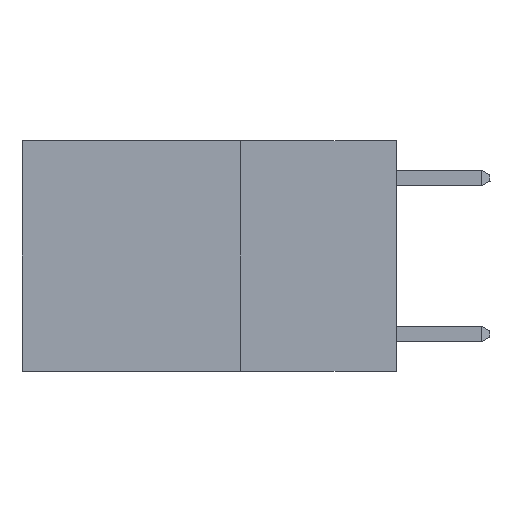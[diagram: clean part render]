
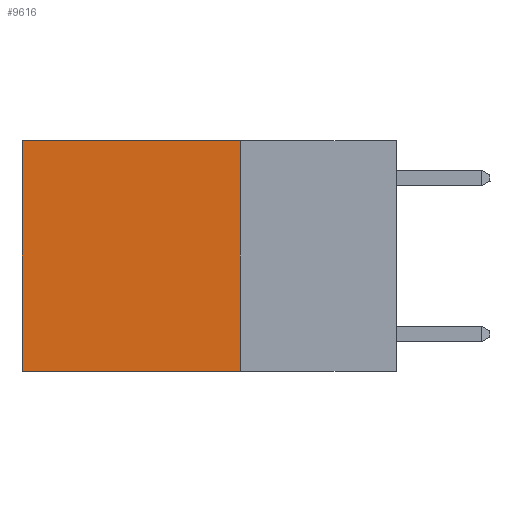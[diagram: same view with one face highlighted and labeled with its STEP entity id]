
A CAD part, left-side view. The second image highlights one B-rep face of the part: STEP entity #9616.
In plain terms, the highlighted planar face has unit normal (-1, 0, 0).
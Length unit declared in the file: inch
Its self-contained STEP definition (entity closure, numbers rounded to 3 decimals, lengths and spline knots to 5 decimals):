
#2076 = VERTEX_POINT ( 'NONE', #5100 ) ;
#2404 = VECTOR ( 'NONE', #7611, 39.37008 ) ;
#2721 = CARTESIAN_POINT ( 'NONE',  ( 0.2625, 0.25, 0. ) ) ;
#4051 = EDGE_CURVE ( 'NONE', #2076, #20402, #18333, .T. ) ;
#4204 = VECTOR ( 'NONE', #20596, 39.37008 ) ;
#4466 = CARTESIAN_POINT ( 'NONE',  ( 0.2625, 0.25, -0.37 ) ) ;
#4641 = DIRECTION ( 'NONE',  ( 0., 0., -1. ) ) ;
#5100 = CARTESIAN_POINT ( 'NONE',  ( 0.2625, 0.25, 0. ) ) ;
#5956 = DIRECTION ( 'NONE',  ( 0., 1., 0. ) ) ;
#6294 = CARTESIAN_POINT ( 'NONE',  ( 0.2625, 0.6, 0. ) ) ;
#7611 = DIRECTION ( 'NONE',  ( 0., 1., 0. ) ) ;
#8493 = EDGE_CURVE ( 'NONE', #20402, #16461, #10672, .T. ) ;
#8768 = VERTEX_POINT ( 'NONE', #4466 ) ;
#9222 = EDGE_CURVE ( 'NONE', #2076, #8768, #19776, .T. ) ;
#9415 = CARTESIAN_POINT ( 'NONE',  ( 0.2625, 0.25, 0. ) ) ;
#9616 = ADVANCED_FACE ( 'NONE', ( #20385 ), #10664, .F. ) ;
#10664 = PLANE ( 'NONE',  #22278 ) ;
#10672 = LINE ( 'NONE', #18701, #4204 ) ;
#11073 = CARTESIAN_POINT ( 'NONE',  ( 0.2625, 0.25, 0. ) ) ;
#11744 = CARTESIAN_POINT ( 'NONE',  ( 0.2625, 0.6, -0.37 ) ) ;
#11941 = ORIENTED_EDGE ( 'NONE', *, *, #4051, .T. ) ;
#12395 = VECTOR ( 'NONE', #4641, 39.37008 ) ;
#12465 = ORIENTED_EDGE ( 'NONE', *, *, #9222, .F. ) ;
#13559 = EDGE_CURVE ( 'NONE', #8768, #16461, #19141, .T. ) ;
#13970 = EDGE_LOOP ( 'NONE', ( #20365, #23858, #12465, #11941 ) ) ;
#14142 = VECTOR ( 'NONE', #5956, 39.37008 ) ;
#16461 = VERTEX_POINT ( 'NONE', #11744 ) ;
#18333 = LINE ( 'NONE', #9415, #2404 ) ;
#18701 = CARTESIAN_POINT ( 'NONE',  ( 0.2625, 0.6, 0. ) ) ;
#18943 = CARTESIAN_POINT ( 'NONE',  ( 0.2625, 0.25, -0.37 ) ) ;
#19141 = LINE ( 'NONE', #18943, #14142 ) ;
#19776 = LINE ( 'NONE', #2721, #12395 ) ;
#20283 = DIRECTION ( 'NONE',  ( 0., 0., -1. ) ) ;
#20365 = ORIENTED_EDGE ( 'NONE', *, *, #8493, .T. ) ;
#20385 = FACE_OUTER_BOUND ( 'NONE', #13970, .T. ) ;
#20402 = VERTEX_POINT ( 'NONE', #6294 ) ;
#20596 = DIRECTION ( 'NONE',  ( 0., 0., -1. ) ) ;
#20808 = DIRECTION ( 'NONE',  ( 1., 0., 0. ) ) ;
#22278 = AXIS2_PLACEMENT_3D ( 'NONE', #11073, #20808, #20283 ) ;
#23858 = ORIENTED_EDGE ( 'NONE', *, *, #13559, .F. ) ;
